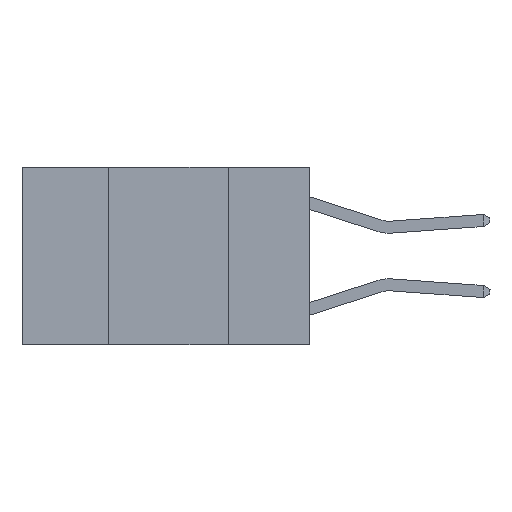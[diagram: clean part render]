
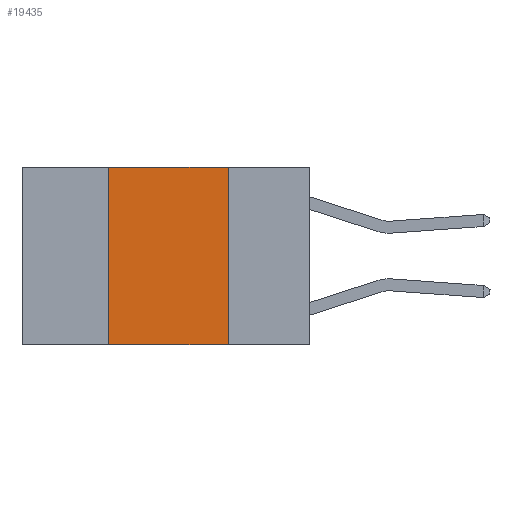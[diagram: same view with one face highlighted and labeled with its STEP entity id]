
A CAD part, left-side view. The second image highlights one B-rep face of the part: STEP entity #19435.
In plain terms, the highlighted planar face has unit normal (-1, 0, 0).
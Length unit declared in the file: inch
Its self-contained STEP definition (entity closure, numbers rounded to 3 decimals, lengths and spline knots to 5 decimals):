
#853 = EDGE_CURVE ( 'NONE', #16615, #15404, #7819, .T. ) ;
#2881 = DIRECTION ( 'NONE',  ( 0., 0., 1. ) ) ;
#3245 = LINE ( 'NONE', #9515, #14110 ) ;
#3392 = EDGE_CURVE ( 'NONE', #5794, #16615, #6735, .T. ) ;
#4286 = DIRECTION ( 'NONE',  ( 0., 0., -1. ) ) ;
#4834 = LINE ( 'NONE', #26173, #23723 ) ;
#4961 = CARTESIAN_POINT ( 'NONE',  ( 0., 0.42, 0. ) ) ;
#5155 = DIRECTION ( 'NONE',  ( 0., 0., -1. ) ) ;
#5287 = VECTOR ( 'NONE', #2881, 39.37008 ) ;
#5794 = VERTEX_POINT ( 'NONE', #26219 ) ;
#6735 = LINE ( 'NONE', #4961, #5287 ) ;
#7819 = LINE ( 'NONE', #10232, #8870 ) ;
#8870 = VECTOR ( 'NONE', #13942, 39.37008 ) ;
#9515 = CARTESIAN_POINT ( 'NONE',  ( 0., 0.17, 0. ) ) ;
#10232 = CARTESIAN_POINT ( 'NONE',  ( 0., 0.6, 0. ) ) ;
#11060 = CARTESIAN_POINT ( 'NONE',  ( 0., 0.17, 0. ) ) ;
#11506 = DIRECTION ( 'NONE',  ( 0., -1., 0. ) ) ;
#12891 = CARTESIAN_POINT ( 'NONE',  ( 0., 0.6, 0. ) ) ;
#13942 = DIRECTION ( 'NONE',  ( 0., -1., 0. ) ) ;
#14110 = VECTOR ( 'NONE', #5155, 39.37008 ) ;
#14774 = CARTESIAN_POINT ( 'NONE',  ( 0., 0.42, 0. ) ) ;
#15195 = VERTEX_POINT ( 'NONE', #20524 ) ;
#15404 = VERTEX_POINT ( 'NONE', #11060 ) ;
#15769 = AXIS2_PLACEMENT_3D ( 'NONE', #12891, #23027, #4286 ) ;
#16615 = VERTEX_POINT ( 'NONE', #14774 ) ;
#16857 = FACE_OUTER_BOUND ( 'NONE', #25656, .T. ) ;
#18198 = ORIENTED_EDGE ( 'NONE', *, *, #26449, .T. ) ;
#19435 = ADVANCED_FACE ( 'NONE', ( #16857 ), #21121, .F. ) ;
#19969 = ORIENTED_EDGE ( 'NONE', *, *, #3392, .F. ) ;
#20524 = CARTESIAN_POINT ( 'NONE',  ( 0., 0.17, -0.37 ) ) ;
#21121 = PLANE ( 'NONE',  #15769 ) ;
#23027 = DIRECTION ( 'NONE',  ( 1., 0., 0. ) ) ;
#23723 = VECTOR ( 'NONE', #11506, 39.37008 ) ;
#24608 = ORIENTED_EDGE ( 'NONE', *, *, #853, .F. ) ;
#25592 = EDGE_CURVE ( 'NONE', #15404, #15195, #3245, .T. ) ;
#25656 = EDGE_LOOP ( 'NONE', ( #26532, #24608, #19969, #18198 ) ) ;
#26173 = CARTESIAN_POINT ( 'NONE',  ( 0., 0.6, -0.37 ) ) ;
#26219 = CARTESIAN_POINT ( 'NONE',  ( 0., 0.42, -0.37 ) ) ;
#26449 = EDGE_CURVE ( 'NONE', #5794, #15195, #4834, .T. ) ;
#26532 = ORIENTED_EDGE ( 'NONE', *, *, #25592, .F. ) ;
